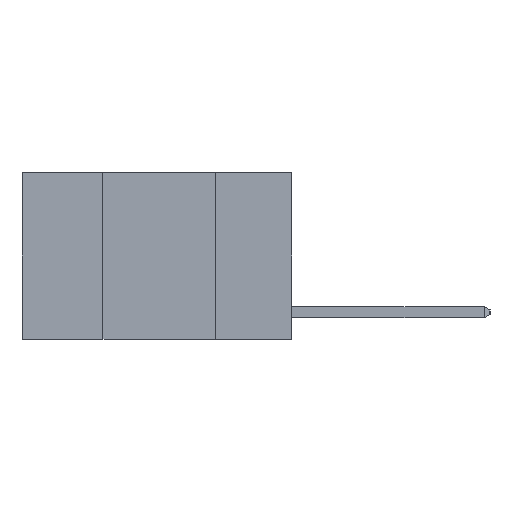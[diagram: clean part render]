
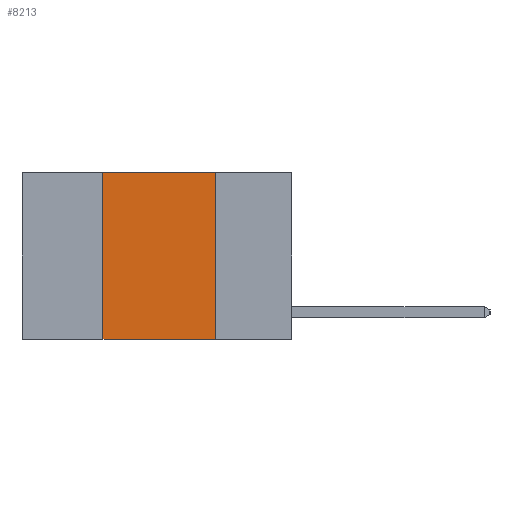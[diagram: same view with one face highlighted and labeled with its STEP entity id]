
A CAD part, left-side view. The second image highlights one B-rep face of the part: STEP entity #8213.
In plain terms, the highlighted planar face has unit normal (-1, 0, 0).
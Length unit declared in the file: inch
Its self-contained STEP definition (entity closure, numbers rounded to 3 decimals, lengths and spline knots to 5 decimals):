
#307 = PLANE ( 'NONE',  #6430 ) ;
#1055 = DIRECTION ( 'NONE',  ( 1., 0., 0. ) ) ;
#1097 = CARTESIAN_POINT ( 'NONE',  ( 0., 0.6, 0. ) ) ;
#1369 = VECTOR ( 'NONE', #7745, 39.37008 ) ;
#1451 = VERTEX_POINT ( 'NONE', #2088 ) ;
#1613 = VERTEX_POINT ( 'NONE', #5593 ) ;
#1686 = CARTESIAN_POINT ( 'NONE',  ( 0., 0.42, 0. ) ) ;
#2013 = EDGE_CURVE ( 'NONE', #1451, #9195, #3297, .T. ) ;
#2019 = CARTESIAN_POINT ( 'NONE',  ( 0., 0.17, 0. ) ) ;
#2088 = CARTESIAN_POINT ( 'NONE',  ( 0., 0.42, 0. ) ) ;
#2132 = VECTOR ( 'NONE', #6136, 39.37008 ) ;
#2934 = FACE_OUTER_BOUND ( 'NONE', #5848, .T. ) ;
#3297 = LINE ( 'NONE', #1097, #1369 ) ;
#3555 = VECTOR ( 'NONE', #6991, 39.37008 ) ;
#3994 = EDGE_CURVE ( 'NONE', #1613, #5905, #4031, .T. ) ;
#4018 = CARTESIAN_POINT ( 'NONE',  ( 0., 0.6, -0.37 ) ) ;
#4031 = LINE ( 'NONE', #4018, #2132 ) ;
#4050 = CARTESIAN_POINT ( 'NONE',  ( 0., 0.17, -0.37 ) ) ;
#4350 = ORIENTED_EDGE ( 'NONE', *, *, #5366, .F. ) ;
#4463 = EDGE_CURVE ( 'NONE', #1613, #1451, #5418, .T. ) ;
#5073 = CARTESIAN_POINT ( 'NONE',  ( 0., 0.17, 0. ) ) ;
#5366 = EDGE_CURVE ( 'NONE', #9195, #5905, #8944, .T. ) ;
#5418 = LINE ( 'NONE', #1686, #5649 ) ;
#5593 = CARTESIAN_POINT ( 'NONE',  ( 0., 0.42, -0.37 ) ) ;
#5649 = VECTOR ( 'NONE', #8004, 39.37008 ) ;
#5848 = EDGE_LOOP ( 'NONE', ( #4350, #6212, #6444, #8313 ) ) ;
#5905 = VERTEX_POINT ( 'NONE', #4050 ) ;
#6032 = DIRECTION ( 'NONE',  ( 0., 0., -1. ) ) ;
#6136 = DIRECTION ( 'NONE',  ( 0., -1., 0. ) ) ;
#6212 = ORIENTED_EDGE ( 'NONE', *, *, #2013, .F. ) ;
#6430 = AXIS2_PLACEMENT_3D ( 'NONE', #7432, #1055, #6032 ) ;
#6444 = ORIENTED_EDGE ( 'NONE', *, *, #4463, .F. ) ;
#6991 = DIRECTION ( 'NONE',  ( 0., 0., -1. ) ) ;
#7432 = CARTESIAN_POINT ( 'NONE',  ( 0., 0.6, 0. ) ) ;
#7745 = DIRECTION ( 'NONE',  ( 0., -1., 0. ) ) ;
#8004 = DIRECTION ( 'NONE',  ( 0., 0., 1. ) ) ;
#8213 = ADVANCED_FACE ( 'NONE', ( #2934 ), #307, .F. ) ;
#8313 = ORIENTED_EDGE ( 'NONE', *, *, #3994, .T. ) ;
#8944 = LINE ( 'NONE', #2019, #3555 ) ;
#9195 = VERTEX_POINT ( 'NONE', #5073 ) ;
